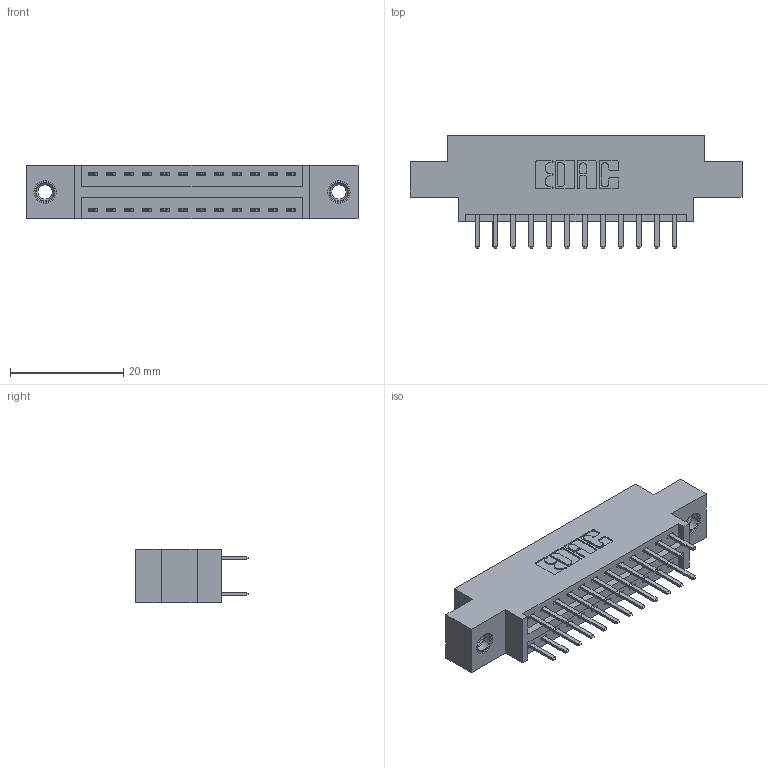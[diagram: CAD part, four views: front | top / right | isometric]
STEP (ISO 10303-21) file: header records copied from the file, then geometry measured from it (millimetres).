
FILE_DESCRIPTION (( 'STEP AP203' ), '1' );
FILE_NAME ('346-024-520-807.STEP', '2022-05-18T22:49:37', ( '' ), ( '' ), 'SwSTEP 2.0', 'SolidWorks 2020', '' );
FILE_SCHEMA (( 'CONFIG_CONTROL_DESIGN' ));
Length unit declared in the file: inch
Products named in the file (4): 346-024-520-807; 345-250-001_345-250-005-103; 345-292-001_345-293-120; 346 Part_0.170 Offset - 0.156 Dia-TI
Assembly tree (27 placements, depth 2):
  346-024-520-807
    346 Part_0.170 Offset - 0.156 Dia-TI
    345-292-001_345-293-120  x24
    345-250-001_345-250-005-103  x2
Bounding box: 58.67 x 20.02 x 9.4 mm (x, y, z)
Volume: 5309.8 mm3; surface area: 7015.7 mm2
Topology: 27 solids, 27 shells, 1530 faces, 4389 edges, 2854 vertices
Faces by surface type: plane 1000, cylinder 514, cone 12, torus 4
Entity records: 13302 total; most frequent: CARTESIAN_POINT 2231, ORIENTED_EDGE 2146, DIRECTION 2031, EDGE_CURVE 1073, LINE 869, VECTOR 869, VERTEX_POINT 708, AXIS2_PLACEMENT_3D 581
